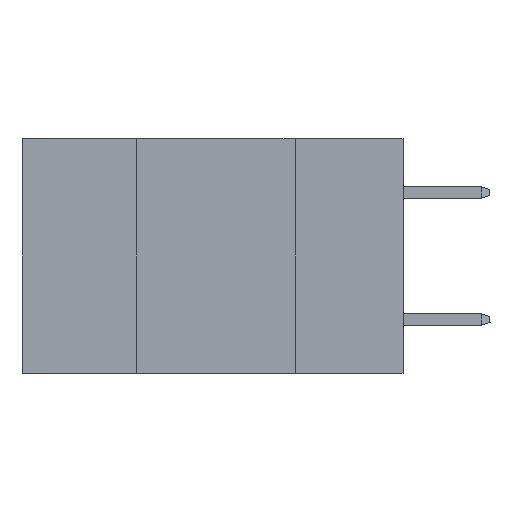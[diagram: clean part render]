
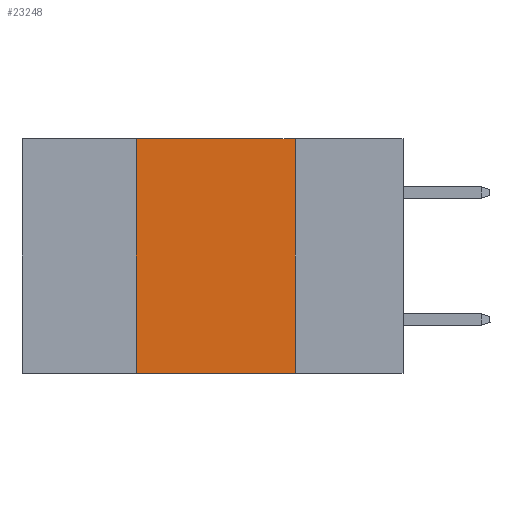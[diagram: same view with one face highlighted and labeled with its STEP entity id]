
A CAD part, left-side view. The second image highlights one B-rep face of the part: STEP entity #23248.
In plain terms, the highlighted planar face has unit normal (-1, 0, 0).
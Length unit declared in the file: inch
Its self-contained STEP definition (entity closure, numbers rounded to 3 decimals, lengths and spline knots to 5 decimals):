
#158 = ORIENTED_EDGE ( 'NONE', *, *, #15177, .F. ) ;
#999 = LINE ( 'NONE', #16529, #9861 ) ;
#1540 = CARTESIAN_POINT ( 'NONE',  ( 0., 0.17, 0. ) ) ;
#2881 = DIRECTION ( 'NONE',  ( 0., 0., -1. ) ) ;
#3237 = DIRECTION ( 'NONE',  ( 0., 0., -1. ) ) ;
#3563 = CARTESIAN_POINT ( 'NONE',  ( 0., 0.42, -0.37 ) ) ;
#4073 = CARTESIAN_POINT ( 'NONE',  ( 0., 0.42, 0. ) ) ;
#5858 = VERTEX_POINT ( 'NONE', #3563 ) ;
#6357 = DIRECTION ( 'NONE',  ( 0., 0., 1. ) ) ;
#6638 = VECTOR ( 'NONE', #3237, 39.37008 ) ;
#7420 = VECTOR ( 'NONE', #6357, 39.37008 ) ;
#8255 = CARTESIAN_POINT ( 'NONE',  ( 0., 0.17, -0.37 ) ) ;
#9129 = PLANE ( 'NONE',  #20107 ) ;
#9276 = DIRECTION ( 'NONE',  ( 1., 0., 0. ) ) ;
#9861 = VECTOR ( 'NONE', #24828, 39.37008 ) ;
#11884 = VERTEX_POINT ( 'NONE', #22316 ) ;
#13604 = CARTESIAN_POINT ( 'NONE',  ( 0., 0.6, 0. ) ) ;
#14517 = EDGE_CURVE ( 'NONE', #5858, #17170, #27462, .T. ) ;
#15177 = EDGE_CURVE ( 'NONE', #17170, #11884, #22211, .T. ) ;
#15180 = DIRECTION ( 'NONE',  ( 0., -1., 0. ) ) ;
#15610 = FACE_OUTER_BOUND ( 'NONE', #20974, .T. ) ;
#16374 = LINE ( 'NONE', #1540, #6638 ) ;
#16425 = VERTEX_POINT ( 'NONE', #8255 ) ;
#16529 = CARTESIAN_POINT ( 'NONE',  ( 0., 0.6, -0.37 ) ) ;
#17162 = ORIENTED_EDGE ( 'NONE', *, *, #27555, .T. ) ;
#17170 = VERTEX_POINT ( 'NONE', #18306 ) ;
#18306 = CARTESIAN_POINT ( 'NONE',  ( 0., 0.42, 0. ) ) ;
#20107 = AXIS2_PLACEMENT_3D ( 'NONE', #26151, #9276, #2881 ) ;
#20373 = ORIENTED_EDGE ( 'NONE', *, *, #25685, .F. ) ;
#20974 = EDGE_LOOP ( 'NONE', ( #20373, #158, #26960, #17162 ) ) ;
#22211 = LINE ( 'NONE', #13604, #24931 ) ;
#22316 = CARTESIAN_POINT ( 'NONE',  ( 0., 0.17, 0. ) ) ;
#23248 = ADVANCED_FACE ( 'NONE', ( #15610 ), #9129, .F. ) ;
#24828 = DIRECTION ( 'NONE',  ( 0., -1., 0. ) ) ;
#24931 = VECTOR ( 'NONE', #15180, 39.37008 ) ;
#25685 = EDGE_CURVE ( 'NONE', #11884, #16425, #16374, .T. ) ;
#26151 = CARTESIAN_POINT ( 'NONE',  ( 0., 0.6, 0. ) ) ;
#26960 = ORIENTED_EDGE ( 'NONE', *, *, #14517, .F. ) ;
#27462 = LINE ( 'NONE', #4073, #7420 ) ;
#27555 = EDGE_CURVE ( 'NONE', #5858, #16425, #999, .T. ) ;
